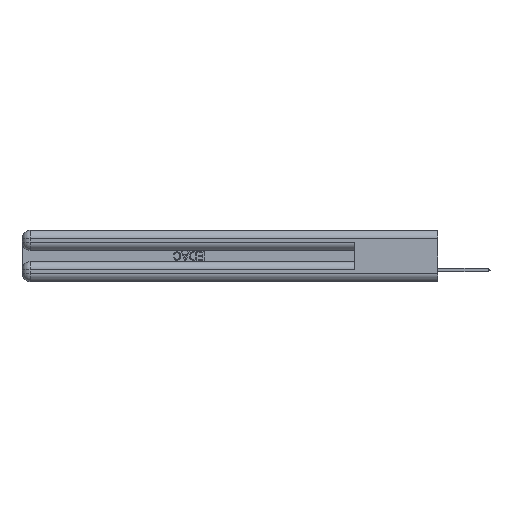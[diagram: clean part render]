
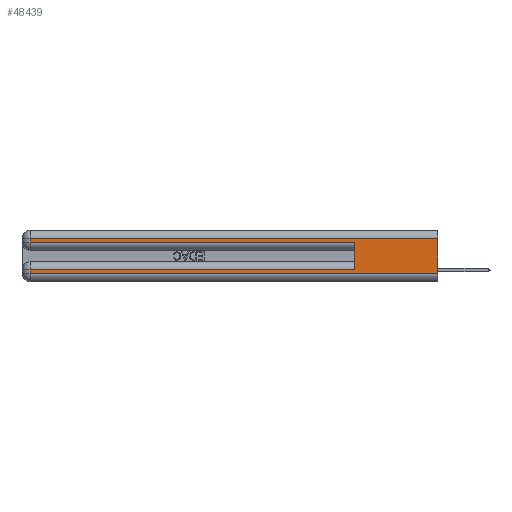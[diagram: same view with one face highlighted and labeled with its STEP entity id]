
A CAD part, left-side view. The second image highlights one B-rep face of the part: STEP entity #48439.
In plain terms, the highlighted planar face has unit normal (-1, 0, 0).
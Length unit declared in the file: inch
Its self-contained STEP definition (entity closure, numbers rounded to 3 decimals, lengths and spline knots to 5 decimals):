
#1388 = EDGE_CURVE ( 'NONE', #24157, #36532, #54482, .T. ) ;
#2216 = LINE ( 'NONE', #6457, #5468 ) ;
#3776 = LINE ( 'NONE', #13462, #47281 ) ;
#3935 = CARTESIAN_POINT ( 'NONE',  ( 0., 2.94, 0.31 ) ) ;
#4138 = CARTESIAN_POINT ( 'NONE',  ( 0., 0., 0.31 ) ) ;
#5236 = VERTEX_POINT ( 'NONE', #3935 ) ;
#5468 = VECTOR ( 'NONE', #53421, 39.37008 ) ;
#6427 = VERTEX_POINT ( 'NONE', #14949 ) ;
#6457 = CARTESIAN_POINT ( 'NONE',  ( 0., 0., 0.06 ) ) ;
#7945 = CARTESIAN_POINT ( 'NONE',  ( 0., 0., 0.37 ) ) ;
#8232 = VERTEX_POINT ( 'NONE', #10848 ) ;
#10476 = LINE ( 'NONE', #7945, #33808 ) ;
#10848 = CARTESIAN_POINT ( 'NONE',  ( 0., 2.94, 0.085 ) ) ;
#10934 = EDGE_CURVE ( 'NONE', #30149, #45611, #10476, .T. ) ;
#12592 = ORIENTED_EDGE ( 'NONE', *, *, #10934, .F. ) ;
#12673 = DIRECTION ( 'NONE',  ( 0., 0., 1. ) ) ;
#13022 = EDGE_CURVE ( 'NONE', #24157, #8232, #24214, .T. ) ;
#13118 = EDGE_CURVE ( 'NONE', #5236, #14414, #13505, .T. ) ;
#13462 = CARTESIAN_POINT ( 'NONE',  ( 0., 0., 0.285 ) ) ;
#13505 = LINE ( 'NONE', #35621, #36795 ) ;
#14414 = VERTEX_POINT ( 'NONE', #45332 ) ;
#14468 = DIRECTION ( 'NONE',  ( 0., 0., -1. ) ) ;
#14949 = CARTESIAN_POINT ( 'NONE',  ( 0., 2.94, 0.06 ) ) ;
#19637 = LINE ( 'NONE', #36665, #49394 ) ;
#20801 = ORIENTED_EDGE ( 'NONE', *, *, #24552, .T. ) ;
#21720 = ORIENTED_EDGE ( 'NONE', *, *, #13118, .T. ) ;
#22321 = CARTESIAN_POINT ( 'NONE',  ( 0., 0.6, 0.085 ) ) ;
#22922 = ORIENTED_EDGE ( 'NONE', *, *, #13022, .T. ) ;
#24157 = VERTEX_POINT ( 'NONE', #22321 ) ;
#24214 = LINE ( 'NONE', #40221, #34723 ) ;
#24552 = EDGE_CURVE ( 'NONE', #8232, #6427, #38593, .T. ) ;
#24828 = DIRECTION ( 'NONE',  ( 0., 0., -1. ) ) ;
#25832 = DIRECTION ( 'NONE',  ( 0., 0., -1. ) ) ;
#26177 = PLANE ( 'NONE',  #31568 ) ;
#27233 = CARTESIAN_POINT ( 'NONE',  ( 0., 0., 0.06 ) ) ;
#30149 = VERTEX_POINT ( 'NONE', #4138 ) ;
#31568 = AXIS2_PLACEMENT_3D ( 'NONE', #35007, #51590, #38893 ) ;
#32314 = CARTESIAN_POINT ( 'NONE',  ( 0., 0.6, 0.285 ) ) ;
#32485 = CARTESIAN_POINT ( 'NONE',  ( 0., 0.6, 0.145 ) ) ;
#33808 = VECTOR ( 'NONE', #25832, 39.37008 ) ;
#34454 = EDGE_LOOP ( 'NONE', ( #12592, #53365, #21720, #52190, #38706, #22922, #20801, #50554 ) ) ;
#34723 = VECTOR ( 'NONE', #48233, 39.37008 ) ;
#34906 = EDGE_CURVE ( 'NONE', #14414, #36532, #3776, .T. ) ;
#35007 = CARTESIAN_POINT ( 'NONE',  ( 0., 0., 0.37 ) ) ;
#35621 = CARTESIAN_POINT ( 'NONE',  ( 0., 2.94, 0.37 ) ) ;
#36532 = VERTEX_POINT ( 'NONE', #32314 ) ;
#36665 = CARTESIAN_POINT ( 'NONE',  ( 0., 0., 0.31 ) ) ;
#36795 = VECTOR ( 'NONE', #14468, 39.37008 ) ;
#38593 = LINE ( 'NONE', #45872, #48426 ) ;
#38706 = ORIENTED_EDGE ( 'NONE', *, *, #1388, .F. ) ;
#38893 = DIRECTION ( 'NONE',  ( 0., 0., -1. ) ) ;
#40221 = CARTESIAN_POINT ( 'NONE',  ( 0., 0., 0.085 ) ) ;
#41544 = EDGE_CURVE ( 'NONE', #6427, #45611, #2216, .T. ) ;
#43066 = FACE_OUTER_BOUND ( 'NONE', #34454, .T. ) ;
#45332 = CARTESIAN_POINT ( 'NONE',  ( 0., 2.94, 0.285 ) ) ;
#45611 = VERTEX_POINT ( 'NONE', #27233 ) ;
#45872 = CARTESIAN_POINT ( 'NONE',  ( 0., 2.94, 0.37 ) ) ;
#47281 = VECTOR ( 'NONE', #47615, 39.37008 ) ;
#47615 = DIRECTION ( 'NONE',  ( 0., -1., 0. ) ) ;
#48233 = DIRECTION ( 'NONE',  ( 0., 1., 0. ) ) ;
#48426 = VECTOR ( 'NONE', #24828, 39.37008 ) ;
#48430 = VECTOR ( 'NONE', #12673, 39.37008 ) ;
#48439 = ADVANCED_FACE ( 'NONE', ( #43066 ), #26177, .F. ) ;
#49394 = VECTOR ( 'NONE', #54032, 39.37008 ) ;
#50554 = ORIENTED_EDGE ( 'NONE', *, *, #41544, .T. ) ;
#51576 = EDGE_CURVE ( 'NONE', #30149, #5236, #19637, .T. ) ;
#51590 = DIRECTION ( 'NONE',  ( 1., 0., 0. ) ) ;
#52190 = ORIENTED_EDGE ( 'NONE', *, *, #34906, .T. ) ;
#53365 = ORIENTED_EDGE ( 'NONE', *, *, #51576, .T. ) ;
#53421 = DIRECTION ( 'NONE',  ( 0., -1., 0. ) ) ;
#54032 = DIRECTION ( 'NONE',  ( 0., 1., 0. ) ) ;
#54482 = LINE ( 'NONE', #32485, #48430 ) ;
